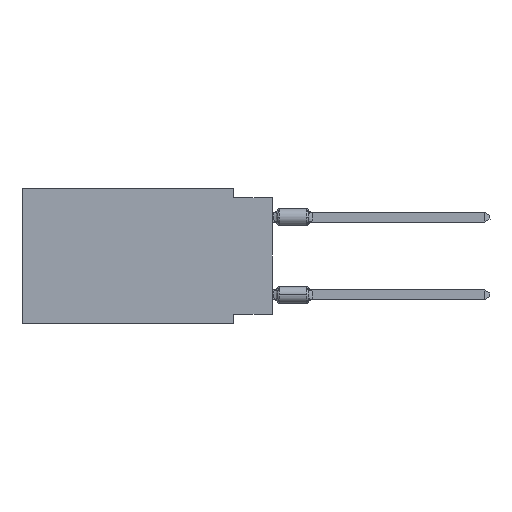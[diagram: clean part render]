
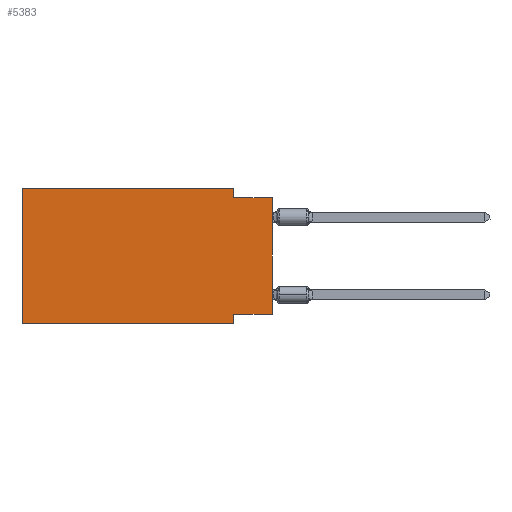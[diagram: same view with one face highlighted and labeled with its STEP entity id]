
A CAD part, left-side view. The second image highlights one B-rep face of the part: STEP entity #5383.
In plain terms, the highlighted planar face has unit normal (-1, 0, 0).
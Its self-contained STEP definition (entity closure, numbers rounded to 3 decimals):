
#264 = LINE ( 'NONE', #11259, #14187 ) ;
#438 = CARTESIAN_POINT ( 'NONE',  ( 0., 16.383, 0. ) ) ;
#850 = VERTEX_POINT ( 'NONE', #9523 ) ;
#1093 = CARTESIAN_POINT ( 'NONE',  ( 0., 0., 0. ) ) ;
#1446 = LINE ( 'NONE', #9110, #3521 ) ;
#1507 = VECTOR ( 'NONE', #19315, 1000. ) ;
#1735 = ORIENTED_EDGE ( 'NONE', *, *, #9346, .F. ) ;
#2104 = VECTOR ( 'NONE', #8900, 1000. ) ;
#2216 = EDGE_CURVE ( 'NONE', #15908, #9574, #1446, .T. ) ;
#2550 = CARTESIAN_POINT ( 'NONE',  ( 0., 16.383, 0. ) ) ;
#2738 = FACE_OUTER_BOUND ( 'NONE', #15242, .T. ) ;
#2979 = EDGE_CURVE ( 'NONE', #12481, #13186, #11436, .T. ) ;
#3473 = LINE ( 'NONE', #16784, #11283 ) ;
#3521 = VECTOR ( 'NONE', #18057, 1000. ) ;
#3654 = CARTESIAN_POINT ( 'NONE',  ( 0., 0., -0.635 ) ) ;
#3944 = VERTEX_POINT ( 'NONE', #12279 ) ;
#4141 = DIRECTION ( 'NONE',  ( 1., 0., 0. ) ) ;
#4469 = ORIENTED_EDGE ( 'NONE', *, *, #18619, .F. ) ;
#4630 = DIRECTION ( 'NONE',  ( 0., -1., 0. ) ) ;
#4740 = LINE ( 'NONE', #438, #19324 ) ;
#5095 = CARTESIAN_POINT ( 'NONE',  ( 0., 0., -0.635 ) ) ;
#5283 = DIRECTION ( 'NONE',  ( 0., -1., 0. ) ) ;
#5383 = ADVANCED_FACE ( 'NONE', ( #2738 ), #8913, .F. ) ;
#6467 = LINE ( 'NONE', #12513, #16433 ) ;
#6911 = DIRECTION ( 'NONE',  ( 0., 0., 1. ) ) ;
#8498 = CARTESIAN_POINT ( 'NONE',  ( 0., 2.54, -8.89 ) ) ;
#8606 = LINE ( 'NONE', #14836, #2104 ) ;
#8900 = DIRECTION ( 'NONE',  ( 0., 0., -1. ) ) ;
#8913 = PLANE ( 'NONE',  #15840 ) ;
#9110 = CARTESIAN_POINT ( 'NONE',  ( 0., 16.383, -8.89 ) ) ;
#9346 = EDGE_CURVE ( 'NONE', #10357, #850, #4740, .T. ) ;
#9523 = CARTESIAN_POINT ( 'NONE',  ( 0., 2.54, 0. ) ) ;
#9574 = VERTEX_POINT ( 'NONE', #8498 ) ;
#10052 = VECTOR ( 'NONE', #5283, 1000. ) ;
#10357 = VERTEX_POINT ( 'NONE', #15496 ) ;
#10858 = EDGE_CURVE ( 'NONE', #18339, #9574, #6467, .T. ) ;
#11029 = DIRECTION ( 'NONE',  ( 0., 0., -1. ) ) ;
#11259 = CARTESIAN_POINT ( 'NONE',  ( 0., 16.383, 0. ) ) ;
#11283 = VECTOR ( 'NONE', #18477, 1000. ) ;
#11436 = LINE ( 'NONE', #1093, #1507 ) ;
#12279 = CARTESIAN_POINT ( 'NONE',  ( 0., 2.54, -0.635 ) ) ;
#12481 = VERTEX_POINT ( 'NONE', #14511 ) ;
#12513 = CARTESIAN_POINT ( 'NONE',  ( 0., 2.54, -8.89 ) ) ;
#13186 = VERTEX_POINT ( 'NONE', #3654 ) ;
#13360 = ORIENTED_EDGE ( 'NONE', *, *, #19253, .F. ) ;
#13678 = ORIENTED_EDGE ( 'NONE', *, *, #10858, .F. ) ;
#13847 = EDGE_CURVE ( 'NONE', #850, #3944, #8606, .T. ) ;
#14187 = VECTOR ( 'NONE', #6911, 1000. ) ;
#14370 = EDGE_CURVE ( 'NONE', #12481, #18339, #3473, .T. ) ;
#14511 = CARTESIAN_POINT ( 'NONE',  ( 0., 0., -8.255 ) ) ;
#14836 = CARTESIAN_POINT ( 'NONE',  ( 0., 2.54, 0. ) ) ;
#15242 = EDGE_LOOP ( 'NONE', ( #17222, #4469, #16595, #1735, #13360, #17007, #13678, #17574 ) ) ;
#15496 = CARTESIAN_POINT ( 'NONE',  ( 0., 16.383, 0. ) ) ;
#15840 = AXIS2_PLACEMENT_3D ( 'NONE', #2550, #4141, #17937 ) ;
#15908 = VERTEX_POINT ( 'NONE', #16302 ) ;
#16221 = CARTESIAN_POINT ( 'NONE',  ( 0., 2.54, -8.255 ) ) ;
#16302 = CARTESIAN_POINT ( 'NONE',  ( 0., 16.383, -8.89 ) ) ;
#16433 = VECTOR ( 'NONE', #11029, 1000. ) ;
#16595 = ORIENTED_EDGE ( 'NONE', *, *, #13847, .F. ) ;
#16784 = CARTESIAN_POINT ( 'NONE',  ( 0., 0., -8.255 ) ) ;
#17007 = ORIENTED_EDGE ( 'NONE', *, *, #2216, .T. ) ;
#17107 = LINE ( 'NONE', #5095, #10052 ) ;
#17222 = ORIENTED_EDGE ( 'NONE', *, *, #2979, .T. ) ;
#17574 = ORIENTED_EDGE ( 'NONE', *, *, #14370, .F. ) ;
#17937 = DIRECTION ( 'NONE',  ( 0., 0., -1. ) ) ;
#18057 = DIRECTION ( 'NONE',  ( 0., -1., 0. ) ) ;
#18339 = VERTEX_POINT ( 'NONE', #16221 ) ;
#18477 = DIRECTION ( 'NONE',  ( 0., 1., 0. ) ) ;
#18619 = EDGE_CURVE ( 'NONE', #3944, #13186, #17107, .T. ) ;
#19253 = EDGE_CURVE ( 'NONE', #15908, #10357, #264, .T. ) ;
#19315 = DIRECTION ( 'NONE',  ( 0., 0., 1. ) ) ;
#19324 = VECTOR ( 'NONE', #4630, 1000. ) ;
